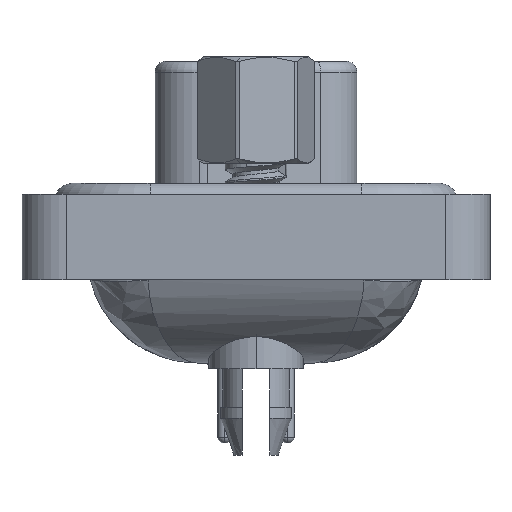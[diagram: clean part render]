
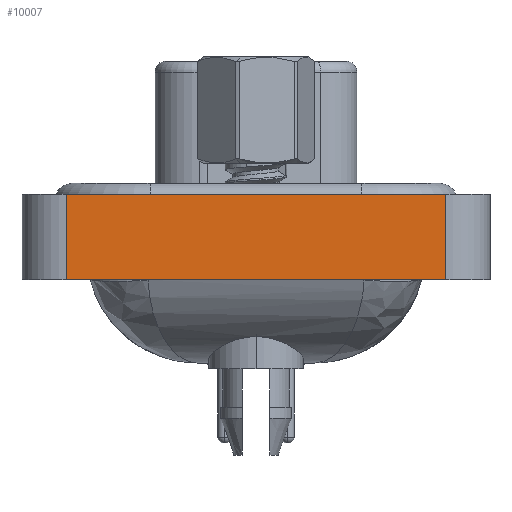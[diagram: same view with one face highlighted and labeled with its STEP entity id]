
A CAD part, left-side view. The second image highlights one B-rep face of the part: STEP entity #10007.
In plain terms, the highlighted planar face has unit normal (-1, 0, 0).
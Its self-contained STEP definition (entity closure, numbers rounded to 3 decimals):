
#2059 = CARTESIAN_POINT ( 'NONE',  ( -7.25, -8.55, -3.35 ) ) ;
#2095 = VECTOR ( 'NONE', #15004, 1000. ) ;
#2119 = CARTESIAN_POINT ( 'NONE',  ( -7.25, -8.55, -3.35 ) ) ;
#2740 = CARTESIAN_POINT ( 'NONE',  ( -7.25, 8.55, -3.35 ) ) ;
#2756 = AXIS2_PLACEMENT_3D ( 'NONE', #2932, #18950, #4502 ) ;
#2932 = CARTESIAN_POINT ( 'NONE',  ( -7.25, -8.55, -3.35 ) ) ;
#3007 = DIRECTION ( 'NONE',  ( 0., -1., 0. ) ) ;
#3152 = ORIENTED_EDGE ( 'NONE', *, *, #18665, .F. ) ;
#4358 = CARTESIAN_POINT ( 'NONE',  ( -7.25, 8.55, 0.5 ) ) ;
#4502 = DIRECTION ( 'NONE',  ( 0., 0., 1. ) ) ;
#5506 = VERTEX_POINT ( 'NONE', #2119 ) ;
#5569 = LINE ( 'NONE', #2740, #20828 ) ;
#5735 = VECTOR ( 'NONE', #12575, 1000. ) ;
#6672 = ORIENTED_EDGE ( 'NONE', *, *, #14763, .T. ) ;
#7274 = EDGE_CURVE ( 'NONE', #5506, #14509, #14146, .T. ) ;
#7658 = FACE_OUTER_BOUND ( 'NONE', #10173, .T. ) ;
#7736 = LINE ( 'NONE', #20612, #20844 ) ;
#8004 = CARTESIAN_POINT ( 'NONE',  ( -7.25, 8.55, -3.35 ) ) ;
#8109 = EDGE_CURVE ( 'NONE', #16902, #14509, #7736, .T. ) ;
#9417 = CARTESIAN_POINT ( 'NONE',  ( -7.25, -8.55, -3.35 ) ) ;
#10007 = ADVANCED_FACE ( 'NONE', ( #7658 ), #14075, .T. ) ;
#10173 = EDGE_LOOP ( 'NONE', ( #17295, #18963, #3152, #6672 ) ) ;
#10741 = VERTEX_POINT ( 'NONE', #8004 ) ;
#12050 = LINE ( 'NONE', #2059, #2095 ) ;
#12575 = DIRECTION ( 'NONE',  ( 0., 0., 1. ) ) ;
#14075 = PLANE ( 'NONE',  #2756 ) ;
#14146 = LINE ( 'NONE', #9417, #5735 ) ;
#14509 = VERTEX_POINT ( 'NONE', #18768 ) ;
#14763 = EDGE_CURVE ( 'NONE', #10741, #5506, #12050, .T. ) ;
#15004 = DIRECTION ( 'NONE',  ( 0., -1., 0. ) ) ;
#16902 = VERTEX_POINT ( 'NONE', #4358 ) ;
#17295 = ORIENTED_EDGE ( 'NONE', *, *, #7274, .T. ) ;
#18655 = DIRECTION ( 'NONE',  ( 0., 0., 1. ) ) ;
#18665 = EDGE_CURVE ( 'NONE', #10741, #16902, #5569, .T. ) ;
#18768 = CARTESIAN_POINT ( 'NONE',  ( -7.25, -8.55, 0.5 ) ) ;
#18950 = DIRECTION ( 'NONE',  ( -1., 0., 0. ) ) ;
#18963 = ORIENTED_EDGE ( 'NONE', *, *, #8109, .F. ) ;
#20612 = CARTESIAN_POINT ( 'NONE',  ( -7.25, -8.55, 0.5 ) ) ;
#20828 = VECTOR ( 'NONE', #18655, 1000. ) ;
#20844 = VECTOR ( 'NONE', #3007, 1000. ) ;
